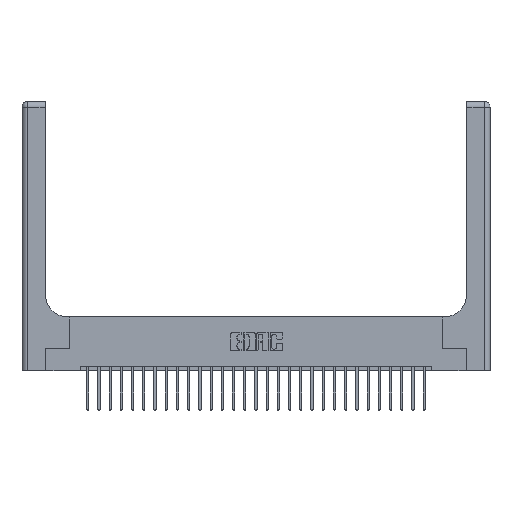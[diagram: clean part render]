
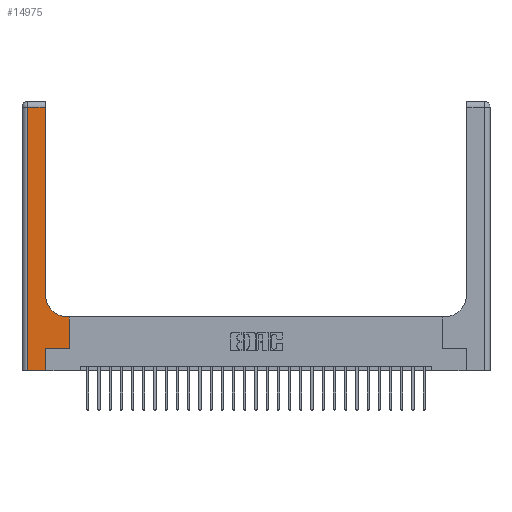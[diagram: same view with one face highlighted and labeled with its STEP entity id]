
A CAD part, top view. The second image highlights one B-rep face of the part: STEP entity #14975.
In plain terms, the highlighted planar face has unit normal (0, 0, 1).
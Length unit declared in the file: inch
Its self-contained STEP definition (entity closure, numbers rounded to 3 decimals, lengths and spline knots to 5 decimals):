
#505 = VERTEX_POINT ( 'NONE', #13647 ) ;
#1166 = VECTOR ( 'NONE', #5563, 39.37008 ) ;
#1533 = VERTEX_POINT ( 'NONE', #8235 ) ;
#1798 = VECTOR ( 'NONE', #13419, 39.37008 ) ;
#1860 = CARTESIAN_POINT ( 'NONE',  ( 0., 3., 0.37 ) ) ;
#2118 = EDGE_CURVE ( 'NONE', #1533, #10485, #8099, .T. ) ;
#2493 = FACE_OUTER_BOUND ( 'NONE', #21368, .T. ) ;
#2950 = EDGE_CURVE ( 'NONE', #11910, #505, #22965, .T. ) ;
#3077 = VECTOR ( 'NONE', #21442, 39.37008 ) ;
#3568 = DIRECTION ( 'NONE',  ( 0., 1., 0. ) ) ;
#4271 = DIRECTION ( 'NONE',  ( 1., 0., 0. ) ) ;
#5152 = VECTOR ( 'NONE', #11042, 39.37008 ) ;
#5246 = AXIS2_PLACEMENT_3D ( 'NONE', #1860, #18478, #18394 ) ;
#5563 = DIRECTION ( 'NONE',  ( 0., 1., 0. ) ) ;
#5807 = VECTOR ( 'NONE', #17144, 39.37008 ) ;
#6245 = CARTESIAN_POINT ( 'NONE',  ( 0.26, 0.85, 0.37 ) ) ;
#6565 = DIRECTION ( 'NONE',  ( -1., 0., 0. ) ) ;
#6678 = VECTOR ( 'NONE', #10700, 39.37008 ) ;
#6894 = CARTESIAN_POINT ( 'NONE',  ( 0., 2.94, 0.37 ) ) ;
#7667 = CARTESIAN_POINT ( 'NONE',  ( 0.528, 0.25, 0.37 ) ) ;
#7926 = CARTESIAN_POINT ( 'NONE',  ( 0.265, 0.25, 0.37 ) ) ;
#8099 = LINE ( 'NONE', #25112, #5152 ) ;
#8235 = CARTESIAN_POINT ( 'NONE',  ( 0.06, 2.94, 0.37 ) ) ;
#8418 = VECTOR ( 'NONE', #6565, 39.37008 ) ;
#9366 = EDGE_CURVE ( 'NONE', #23614, #16944, #19335, .T. ) ;
#9727 = EDGE_CURVE ( 'NONE', #16944, #1533, #12228, .T. ) ;
#9829 = VERTEX_POINT ( 'NONE', #11274 ) ;
#10141 = ORIENTED_EDGE ( 'NONE', *, *, #16512, .T. ) ;
#10485 = VERTEX_POINT ( 'NONE', #26843 ) ;
#10700 = DIRECTION ( 'NONE',  ( 1., 0., 0. ) ) ;
#10855 = CARTESIAN_POINT ( 'NONE',  ( 0.51, 0.85, 0.37 ) ) ;
#11041 = LINE ( 'NONE', #12945, #8418 ) ;
#11042 = DIRECTION ( 'NONE',  ( 0., -1., 0. ) ) ;
#11274 = CARTESIAN_POINT ( 'NONE',  ( 0.51, 0.6, 0.37 ) ) ;
#11910 = VERTEX_POINT ( 'NONE', #7926 ) ;
#12133 = ORIENTED_EDGE ( 'NONE', *, *, #19814, .T. ) ;
#12228 = LINE ( 'NONE', #6894, #3077 ) ;
#12431 = VECTOR ( 'NONE', #3568, 39.37008 ) ;
#12945 = CARTESIAN_POINT ( 'NONE',  ( 0.26, 0.6, 0.37 ) ) ;
#13419 = DIRECTION ( 'NONE',  ( 0., 1., 0. ) ) ;
#13647 = CARTESIAN_POINT ( 'NONE',  ( 0.528, 0.25, 0.37 ) ) ;
#14164 = EDGE_CURVE ( 'NONE', #16148, #9829, #11041, .T. ) ;
#14424 = ORIENTED_EDGE ( 'NONE', *, *, #26661, .T. ) ;
#14975 = ADVANCED_FACE ( 'NONE', ( #2493 ), #20513, .F. ) ;
#15962 = LINE ( 'NONE', #16194, #12431 ) ;
#16148 = VERTEX_POINT ( 'NONE', #23663 ) ;
#16194 = CARTESIAN_POINT ( 'NONE',  ( 0.265, 0., 0.37 ) ) ;
#16275 = EDGE_CURVE ( 'NONE', #19154, #11910, #15962, .T. ) ;
#16512 = EDGE_CURVE ( 'NONE', #9829, #23614, #23477, .T. ) ;
#16944 = VERTEX_POINT ( 'NONE', #24812 ) ;
#17123 = CARTESIAN_POINT ( 'NONE',  ( 0.26, 3., 0.37 ) ) ;
#17144 = DIRECTION ( 'NONE',  ( 1., 0., 0. ) ) ;
#17481 = LINE ( 'NONE', #21613, #5807 ) ;
#18394 = DIRECTION ( 'NONE',  ( -1., 0., 0. ) ) ;
#18478 = DIRECTION ( 'NONE',  ( 0., 0., -1. ) ) ;
#19154 = VERTEX_POINT ( 'NONE', #26287 ) ;
#19295 = ORIENTED_EDGE ( 'NONE', *, *, #16275, .T. ) ;
#19335 = LINE ( 'NONE', #17123, #1798 ) ;
#19702 = LINE ( 'NONE', #7667, #1166 ) ;
#19814 = EDGE_CURVE ( 'NONE', #505, #16148, #19702, .T. ) ;
#19854 = ORIENTED_EDGE ( 'NONE', *, *, #2118, .T. ) ;
#20513 = PLANE ( 'NONE',  #5246 ) ;
#21044 = CARTESIAN_POINT ( 'NONE',  ( 0.265, 0.25, 0.37 ) ) ;
#21368 = EDGE_LOOP ( 'NONE', ( #22565, #26299, #19854, #14424, #19295, #23466, #12133, #23221, #10141 ) ) ;
#21442 = DIRECTION ( 'NONE',  ( -1., 0., 0. ) ) ;
#21613 = CARTESIAN_POINT ( 'NONE',  ( 0., 0., 0.37 ) ) ;
#22348 = AXIS2_PLACEMENT_3D ( 'NONE', #10855, #25105, #4271 ) ;
#22565 = ORIENTED_EDGE ( 'NONE', *, *, #9366, .T. ) ;
#22965 = LINE ( 'NONE', #21044, #6678 ) ;
#23221 = ORIENTED_EDGE ( 'NONE', *, *, #14164, .T. ) ;
#23466 = ORIENTED_EDGE ( 'NONE', *, *, #2950, .T. ) ;
#23477 = CIRCLE ( 'NONE', #22348, 0.25 ) ;
#23614 = VERTEX_POINT ( 'NONE', #6245 ) ;
#23663 = CARTESIAN_POINT ( 'NONE',  ( 0.528, 0.6, 0.37 ) ) ;
#24812 = CARTESIAN_POINT ( 'NONE',  ( 0.26, 2.94, 0.37 ) ) ;
#25105 = DIRECTION ( 'NONE',  ( 0., 0., -1. ) ) ;
#25112 = CARTESIAN_POINT ( 'NONE',  ( 0.06, 3., 0.37 ) ) ;
#26287 = CARTESIAN_POINT ( 'NONE',  ( 0.265, 0., 0.37 ) ) ;
#26299 = ORIENTED_EDGE ( 'NONE', *, *, #9727, .T. ) ;
#26661 = EDGE_CURVE ( 'NONE', #10485, #19154, #17481, .T. ) ;
#26843 = CARTESIAN_POINT ( 'NONE',  ( 0.06, 0., 0.37 ) ) ;
